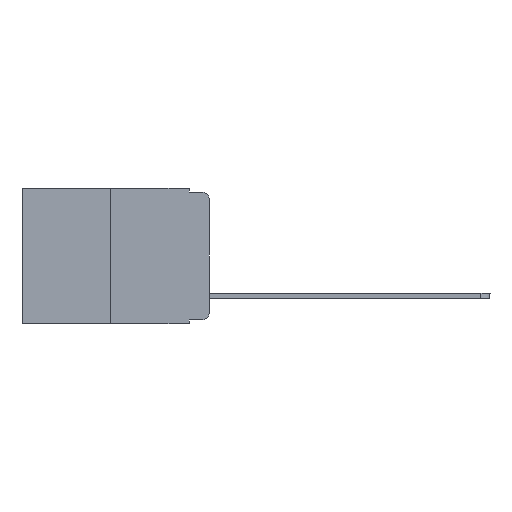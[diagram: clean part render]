
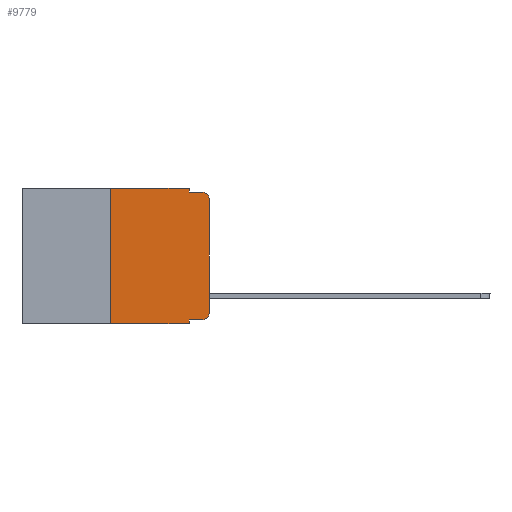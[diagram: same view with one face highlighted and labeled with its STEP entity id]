
A CAD part, left-side view. The second image highlights one B-rep face of the part: STEP entity #9779.
In plain terms, the highlighted planar face has unit normal (-1, 0, 0).
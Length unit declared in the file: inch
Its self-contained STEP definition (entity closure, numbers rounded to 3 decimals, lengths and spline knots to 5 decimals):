
#33 = CARTESIAN_POINT ( 'NONE',  ( 0., 0.473, -0.343 ) ) ;
#59 = EDGE_CURVE ( 'NONE', #1151, #6140, #11702, .T. ) ;
#123 = DIRECTION ( 'NONE',  ( 0., 0., -1. ) ) ;
#443 = FACE_OUTER_BOUND ( 'NONE', #10835, .T. ) ;
#556 = DIRECTION ( 'NONE',  ( 0., -1., 0. ) ) ;
#626 = ORIENTED_EDGE ( 'NONE', *, *, #10898, .T. ) ;
#688 = DIRECTION ( 'NONE',  ( 0., 0., -1. ) ) ;
#896 = CARTESIAN_POINT ( 'NONE',  ( 0., 0.02, -0.313 ) ) ;
#959 = DIRECTION ( 'NONE',  ( -1., 0., 0. ) ) ;
#962 = DIRECTION ( 'NONE',  ( -1., 0., 0. ) ) ;
#1044 = AXIS2_PLACEMENT_3D ( 'NONE', #2148, #962, #5557 ) ;
#1151 = VERTEX_POINT ( 'NONE', #11765 ) ;
#1218 = EDGE_CURVE ( 'NONE', #7206, #8737, #11688, .T. ) ;
#1303 = CARTESIAN_POINT ( 'NONE',  ( 0., 0.051, -0.343 ) ) ;
#1322 = LINE ( 'NONE', #10380, #9283 ) ;
#1395 = CARTESIAN_POINT ( 'NONE',  ( 0., 0.473, 0. ) ) ;
#1666 = VERTEX_POINT ( 'NONE', #1303 ) ;
#1873 = VECTOR ( 'NONE', #5922, 39.37008 ) ;
#2074 = LINE ( 'NONE', #13229, #11038 ) ;
#2104 = CARTESIAN_POINT ( 'NONE',  ( 0., 0.051, -0.333 ) ) ;
#2148 = CARTESIAN_POINT ( 'NONE',  ( 0., 0.02, -0.03 ) ) ;
#2320 = DIRECTION ( 'NONE',  ( 1., 0., 0. ) ) ;
#2777 = CARTESIAN_POINT ( 'NONE',  ( 0., 0.051, -0.01 ) ) ;
#2978 = EDGE_CURVE ( 'NONE', #5555, #8897, #13596, .T. ) ;
#3083 = VERTEX_POINT ( 'NONE', #4010 ) ;
#3389 = CARTESIAN_POINT ( 'NONE',  ( 0., 0.02, -0.01 ) ) ;
#3476 = AXIS2_PLACEMENT_3D ( 'NONE', #12484, #2320, #14121 ) ;
#3506 = ORIENTED_EDGE ( 'NONE', *, *, #11158, .F. ) ;
#3902 = VECTOR ( 'NONE', #13136, 39.37008 ) ;
#4010 = CARTESIAN_POINT ( 'NONE',  ( 0., 0., -0.03 ) ) ;
#4456 = EDGE_CURVE ( 'NONE', #11416, #1666, #1322, .T. ) ;
#4533 = CARTESIAN_POINT ( 'NONE',  ( 0., 0.25, 0. ) ) ;
#4604 = CIRCLE ( 'NONE', #1044, 0.02 ) ;
#5030 = CARTESIAN_POINT ( 'NONE',  ( 0., 0.25, 0. ) ) ;
#5476 = DIRECTION ( 'NONE',  ( 0., 0., -1. ) ) ;
#5555 = VERTEX_POINT ( 'NONE', #10177 ) ;
#5557 = DIRECTION ( 'NONE',  ( 0., 0., -1. ) ) ;
#5922 = DIRECTION ( 'NONE',  ( 0., -1., 0. ) ) ;
#6009 = VECTOR ( 'NONE', #556, 39.37008 ) ;
#6140 = VERTEX_POINT ( 'NONE', #11247 ) ;
#6239 = LINE ( 'NONE', #14269, #10154 ) ;
#6888 = DIRECTION ( 'NONE',  ( 0., 0., 1. ) ) ;
#6979 = EDGE_CURVE ( 'NONE', #3083, #8737, #4604, .T. ) ;
#7047 = ORIENTED_EDGE ( 'NONE', *, *, #1218, .F. ) ;
#7206 = VERTEX_POINT ( 'NONE', #14032 ) ;
#7284 = DIRECTION ( 'NONE',  ( 0., -1., 0. ) ) ;
#7361 = EDGE_CURVE ( 'NONE', #6140, #3083, #12153, .T. ) ;
#7464 = EDGE_CURVE ( 'NONE', #5555, #1666, #12368, .T. ) ;
#8137 = EDGE_CURVE ( 'NONE', #14322, #7206, #2074, .T. ) ;
#8515 = ORIENTED_EDGE ( 'NONE', *, *, #2978, .F. ) ;
#8670 = CARTESIAN_POINT ( 'NONE',  ( 0., 0.051, 0. ) ) ;
#8737 = VERTEX_POINT ( 'NONE', #3389 ) ;
#8859 = ORIENTED_EDGE ( 'NONE', *, *, #7361, .T. ) ;
#8897 = VERTEX_POINT ( 'NONE', #5030 ) ;
#9283 = VECTOR ( 'NONE', #123, 39.37008 ) ;
#9779 = ADVANCED_FACE ( 'NONE', ( #443 ), #11375, .F. ) ;
#10154 = VECTOR ( 'NONE', #7284, 39.37008 ) ;
#10177 = CARTESIAN_POINT ( 'NONE',  ( 0., 0.25, -0.343 ) ) ;
#10380 = CARTESIAN_POINT ( 'NONE',  ( 0., 0.051, 0. ) ) ;
#10835 = EDGE_LOOP ( 'NONE', ( #8859, #12847, #7047, #12185, #3506, #8515, #13888, #11903, #626, #13912 ) ) ;
#10898 = EDGE_CURVE ( 'NONE', #11416, #1151, #6239, .T. ) ;
#11038 = VECTOR ( 'NONE', #688, 39.37008 ) ;
#11158 = EDGE_CURVE ( 'NONE', #8897, #14322, #11570, .T. ) ;
#11247 = CARTESIAN_POINT ( 'NONE',  ( 0., 0., -0.313 ) ) ;
#11375 = PLANE ( 'NONE',  #3476 ) ;
#11416 = VERTEX_POINT ( 'NONE', #2104 ) ;
#11570 = LINE ( 'NONE', #1395, #1873 ) ;
#11688 = LINE ( 'NONE', #2777, #6009 ) ;
#11702 = CIRCLE ( 'NONE', #13598, 0.02 ) ;
#11765 = CARTESIAN_POINT ( 'NONE',  ( 0., 0.02, -0.333 ) ) ;
#11868 = CARTESIAN_POINT ( 'NONE',  ( 0., 0., 0. ) ) ;
#11903 = ORIENTED_EDGE ( 'NONE', *, *, #4456, .F. ) ;
#12153 = LINE ( 'NONE', #11868, #3902 ) ;
#12185 = ORIENTED_EDGE ( 'NONE', *, *, #8137, .F. ) ;
#12368 = LINE ( 'NONE', #33, #12914 ) ;
#12484 = CARTESIAN_POINT ( 'NONE',  ( 0., 0.473, 0. ) ) ;
#12847 = ORIENTED_EDGE ( 'NONE', *, *, #6979, .T. ) ;
#12914 = VECTOR ( 'NONE', #13352, 39.37008 ) ;
#13136 = DIRECTION ( 'NONE',  ( 0., 0., 1. ) ) ;
#13229 = CARTESIAN_POINT ( 'NONE',  ( 0., 0.051, 0. ) ) ;
#13315 = VECTOR ( 'NONE', #6888, 39.37008 ) ;
#13352 = DIRECTION ( 'NONE',  ( 0., -1., 0. ) ) ;
#13596 = LINE ( 'NONE', #4533, #13315 ) ;
#13598 = AXIS2_PLACEMENT_3D ( 'NONE', #896, #959, #5476 ) ;
#13888 = ORIENTED_EDGE ( 'NONE', *, *, #7464, .T. ) ;
#13912 = ORIENTED_EDGE ( 'NONE', *, *, #59, .T. ) ;
#14032 = CARTESIAN_POINT ( 'NONE',  ( 0., 0.051, -0.01 ) ) ;
#14121 = DIRECTION ( 'NONE',  ( 0., 0., -1. ) ) ;
#14269 = CARTESIAN_POINT ( 'NONE',  ( 0., 0.051, -0.333 ) ) ;
#14322 = VERTEX_POINT ( 'NONE', #8670 ) ;
